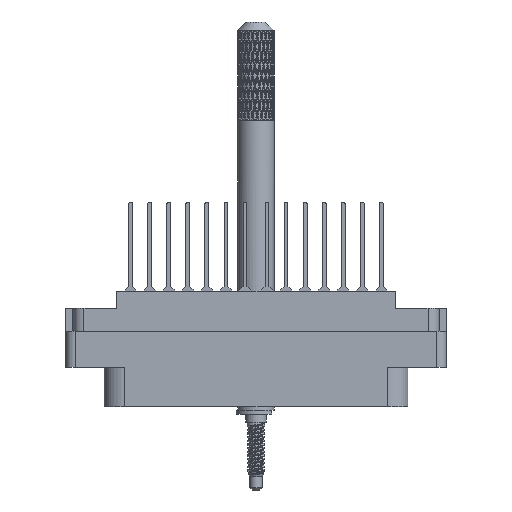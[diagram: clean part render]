
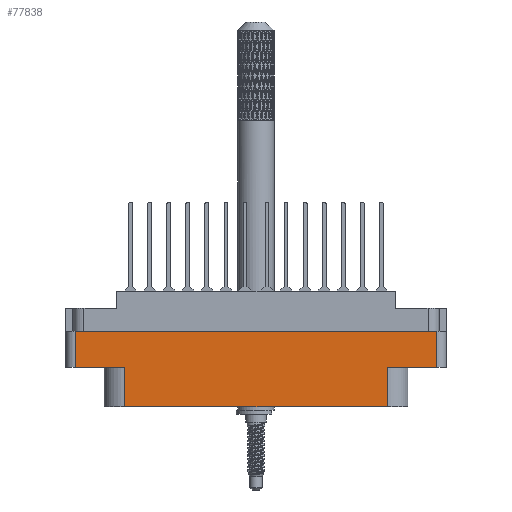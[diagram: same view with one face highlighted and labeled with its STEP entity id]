
A CAD part, front view. The second image highlights one B-rep face of the part: STEP entity #77838.
In plain terms, the highlighted planar face has unit normal (0, -1, 0).
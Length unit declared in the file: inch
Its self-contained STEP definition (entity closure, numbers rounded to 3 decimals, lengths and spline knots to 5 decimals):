
#975 = CARTESIAN_POINT ( 'NONE',  ( 1.2335, -0.438, -0.274 ) ) ;
#1287 = LINE ( 'NONE', #39874, #19320 ) ;
#4169 = EDGE_CURVE ( 'NONE', #81053, #27346, #82184, .T. ) ;
#8544 = VECTOR ( 'NONE', #16933, 39.37008 ) ;
#13695 = ORIENTED_EDGE ( 'NONE', *, *, #4169, .T. ) ;
#14286 = ORIENTED_EDGE ( 'NONE', *, *, #56428, .F. ) ;
#14375 = VERTEX_POINT ( 'NONE', #48605 ) ;
#16860 = EDGE_CURVE ( 'NONE', #79638, #27346, #112908, .T. ) ;
#16886 = CARTESIAN_POINT ( 'NONE',  ( 1.2335, -0.438, -0.52 ) ) ;
#16933 = DIRECTION ( 'NONE',  ( 1., 0., 0. ) ) ;
#18074 = EDGE_CURVE ( 'NONE', #89312, #87654, #52856, .T. ) ;
#18259 = VECTOR ( 'NONE', #81015, 39.37008 ) ;
#19320 = VECTOR ( 'NONE', #101956, 39.37008 ) ;
#20404 = AXIS2_PLACEMENT_3D ( 'NONE', #48222, #91764, #100648 ) ;
#20993 = PLANE ( 'NONE',  #20404 ) ;
#22523 = CARTESIAN_POINT ( 'NONE',  ( -1.2955, -0.438, -0.789 ) ) ;
#23803 = VECTOR ( 'NONE', #66435, 39.37008 ) ;
#27346 = VERTEX_POINT ( 'NONE', #111296 ) ;
#28730 = DIRECTION ( 'NONE',  ( 0., 0., 1. ) ) ;
#29474 = EDGE_CURVE ( 'NONE', #79638, #80562, #48708, .T. ) ;
#30305 = EDGE_CURVE ( 'NONE', #89312, #55742, #1287, .T. ) ;
#31480 = DIRECTION ( 'NONE',  ( 0., 0., 1. ) ) ;
#36051 = ORIENTED_EDGE ( 'NONE', *, *, #29474, .T. ) ;
#36197 = ORIENTED_EDGE ( 'NONE', *, *, #18074, .T. ) ;
#39085 = FACE_OUTER_BOUND ( 'NONE', #79693, .T. ) ;
#39874 = CARTESIAN_POINT ( 'NONE',  ( 0., -0.438, -0.52 ) ) ;
#40184 = CARTESIAN_POINT ( 'NONE',  ( -0.895, -0.438, -0.789 ) ) ;
#40455 = LINE ( 'NONE', #22523, #23803 ) ;
#41636 = EDGE_CURVE ( 'NONE', #87654, #81053, #40455, .T. ) ;
#43358 = LINE ( 'NONE', #114202, #8544 ) ;
#45909 = DIRECTION ( 'NONE',  ( 0., 0., -1. ) ) ;
#48222 = CARTESIAN_POINT ( 'NONE',  ( -1.2955, -0.438, -0.789 ) ) ;
#48605 = CARTESIAN_POINT ( 'NONE',  ( -1.2335, -0.438, -0.274 ) ) ;
#48708 = LINE ( 'NONE', #109235, #76509 ) ;
#49970 = ORIENTED_EDGE ( 'NONE', *, *, #30305, .F. ) ;
#52856 = LINE ( 'NONE', #99070, #91797 ) ;
#55742 = VERTEX_POINT ( 'NONE', #104912 ) ;
#56131 = ORIENTED_EDGE ( 'NONE', *, *, #41636, .T. ) ;
#56428 = EDGE_CURVE ( 'NONE', #14375, #80562, #43358, .T. ) ;
#65246 = CARTESIAN_POINT ( 'NONE',  ( 0.895, -0.438, -0.52 ) ) ;
#66435 = DIRECTION ( 'NONE',  ( 1., 0., 0. ) ) ;
#71155 = LINE ( 'NONE', #108596, #18259 ) ;
#72480 = VECTOR ( 'NONE', #31480, 39.37008 ) ;
#72557 = CARTESIAN_POINT ( 'NONE',  ( 0., -0.438, -0.52 ) ) ;
#76509 = VECTOR ( 'NONE', #28730, 39.37008 ) ;
#77838 = ADVANCED_FACE ( 'NONE', ( #39085 ), #20993, .T. ) ;
#79638 = VERTEX_POINT ( 'NONE', #16886 ) ;
#79693 = EDGE_LOOP ( 'NONE', ( #14286, #81779, #49970, #36197, #56131, #13695, #95835, #36051 ) ) ;
#80562 = VERTEX_POINT ( 'NONE', #975 ) ;
#81015 = DIRECTION ( 'NONE',  ( 0., 0., -1. ) ) ;
#81053 = VERTEX_POINT ( 'NONE', #100883 ) ;
#81147 = DIRECTION ( 'NONE',  ( -1., 0., 0. ) ) ;
#81779 = ORIENTED_EDGE ( 'NONE', *, *, #84349, .T. ) ;
#82184 = LINE ( 'NONE', #65246, #72480 ) ;
#84349 = EDGE_CURVE ( 'NONE', #14375, #55742, #71155, .T. ) ;
#87654 = VERTEX_POINT ( 'NONE', #40184 ) ;
#89312 = VERTEX_POINT ( 'NONE', #94115 ) ;
#91764 = DIRECTION ( 'NONE',  ( 0., -1., 0. ) ) ;
#91797 = VECTOR ( 'NONE', #45909, 39.37008 ) ;
#92019 = VECTOR ( 'NONE', #81147, 39.37008 ) ;
#94115 = CARTESIAN_POINT ( 'NONE',  ( -0.895, -0.438, -0.52 ) ) ;
#95835 = ORIENTED_EDGE ( 'NONE', *, *, #16860, .F. ) ;
#99070 = CARTESIAN_POINT ( 'NONE',  ( -0.895, -0.438, -0.789 ) ) ;
#100648 = DIRECTION ( 'NONE',  ( 0., 0., -1. ) ) ;
#100883 = CARTESIAN_POINT ( 'NONE',  ( 0.895, -0.438, -0.789 ) ) ;
#101956 = DIRECTION ( 'NONE',  ( -1., 0., 0. ) ) ;
#104912 = CARTESIAN_POINT ( 'NONE',  ( -1.2335, -0.438, -0.52 ) ) ;
#108596 = CARTESIAN_POINT ( 'NONE',  ( -1.2335, -0.438, -0.789 ) ) ;
#109235 = CARTESIAN_POINT ( 'NONE',  ( 1.2335, -0.438, -0.789 ) ) ;
#111296 = CARTESIAN_POINT ( 'NONE',  ( 0.895, -0.438, -0.52 ) ) ;
#112908 = LINE ( 'NONE', #72557, #92019 ) ;
#114202 = CARTESIAN_POINT ( 'NONE',  ( 0., -0.438, -0.274 ) ) ;
